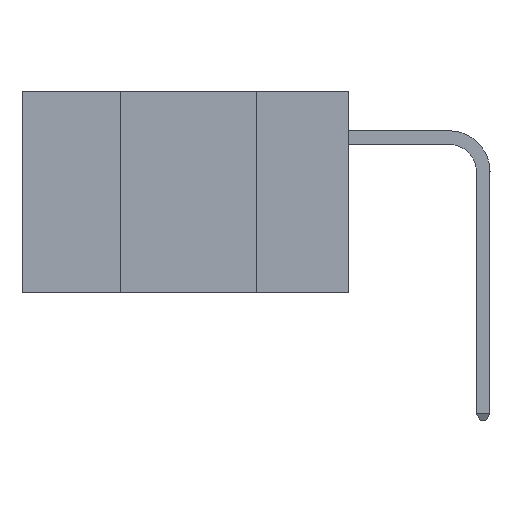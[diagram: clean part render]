
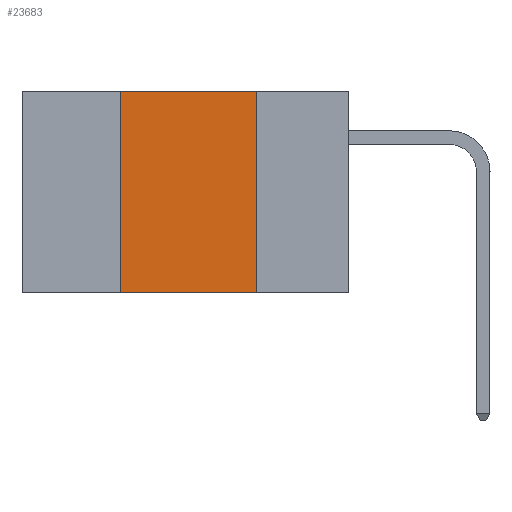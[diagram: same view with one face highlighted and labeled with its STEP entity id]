
A CAD part, left-side view. The second image highlights one B-rep face of the part: STEP entity #23683.
In plain terms, the highlighted planar face has unit normal (-1, 0, 0).
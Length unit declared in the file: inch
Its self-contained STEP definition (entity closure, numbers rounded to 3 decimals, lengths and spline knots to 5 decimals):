
#204 = VERTEX_POINT ( 'NONE', #2561 ) ;
#452 = ORIENTED_EDGE ( 'NONE', *, *, #10934, .F. ) ;
#632 = ORIENTED_EDGE ( 'NONE', *, *, #32111, .T. ) ;
#2561 = CARTESIAN_POINT ( 'NONE',  ( 0., 0.42, -0.37 ) ) ;
#2566 = VECTOR ( 'NONE', #36572, 39.37008 ) ;
#3592 = FACE_OUTER_BOUND ( 'NONE', #33891, .T. ) ;
#3604 = CARTESIAN_POINT ( 'NONE',  ( 0., 0.6, 0. ) ) ;
#3615 = AXIS2_PLACEMENT_3D ( 'NONE', #19665, #13479, #19940 ) ;
#5561 = LINE ( 'NONE', #6328, #33646 ) ;
#6328 = CARTESIAN_POINT ( 'NONE',  ( 0., 0.17, 0. ) ) ;
#6846 = VERTEX_POINT ( 'NONE', #41019 ) ;
#9080 = VECTOR ( 'NONE', #26031, 39.37008 ) ;
#9215 = CARTESIAN_POINT ( 'NONE',  ( 0., 0.42, 0. ) ) ;
#10123 = LINE ( 'NONE', #16905, #2566 ) ;
#10566 = VECTOR ( 'NONE', #21158, 39.37008 ) ;
#10934 = EDGE_CURVE ( 'NONE', #204, #11265, #24606, .T. ) ;
#11265 = VERTEX_POINT ( 'NONE', #9215 ) ;
#13479 = DIRECTION ( 'NONE',  ( 1., 0., 0. ) ) ;
#16905 = CARTESIAN_POINT ( 'NONE',  ( 0., 0.6, -0.37 ) ) ;
#18973 = DIRECTION ( 'NONE',  ( 0., 0., -1. ) ) ;
#19665 = CARTESIAN_POINT ( 'NONE',  ( 0., 0.6, 0. ) ) ;
#19940 = DIRECTION ( 'NONE',  ( 0., 0., -1. ) ) ;
#21158 = DIRECTION ( 'NONE',  ( 0., 0., 1. ) ) ;
#23683 = ADVANCED_FACE ( 'NONE', ( #3592 ), #29059, .F. ) ;
#24417 = ORIENTED_EDGE ( 'NONE', *, *, #39943, .F. ) ;
#24606 = LINE ( 'NONE', #40287, #10566 ) ;
#26031 = DIRECTION ( 'NONE',  ( 0., -1., 0. ) ) ;
#29059 = PLANE ( 'NONE',  #3615 ) ;
#29605 = LINE ( 'NONE', #3604, #9080 ) ;
#31278 = CARTESIAN_POINT ( 'NONE',  ( 0., 0.17, -0.37 ) ) ;
#32111 = EDGE_CURVE ( 'NONE', #204, #34356, #10123, .T. ) ;
#32501 = EDGE_CURVE ( 'NONE', #11265, #6846, #29605, .T. ) ;
#33646 = VECTOR ( 'NONE', #18973, 39.37008 ) ;
#33891 = EDGE_LOOP ( 'NONE', ( #24417, #39398, #452, #632 ) ) ;
#34356 = VERTEX_POINT ( 'NONE', #31278 ) ;
#36572 = DIRECTION ( 'NONE',  ( 0., -1., 0. ) ) ;
#39398 = ORIENTED_EDGE ( 'NONE', *, *, #32501, .F. ) ;
#39943 = EDGE_CURVE ( 'NONE', #6846, #34356, #5561, .T. ) ;
#40287 = CARTESIAN_POINT ( 'NONE',  ( 0., 0.42, 0. ) ) ;
#41019 = CARTESIAN_POINT ( 'NONE',  ( 0., 0.17, 0. ) ) ;
